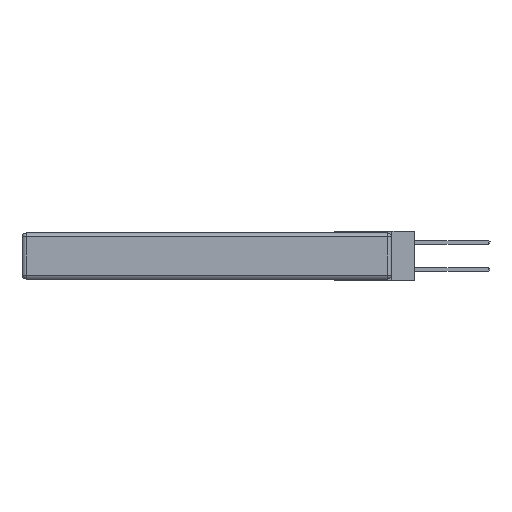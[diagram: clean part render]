
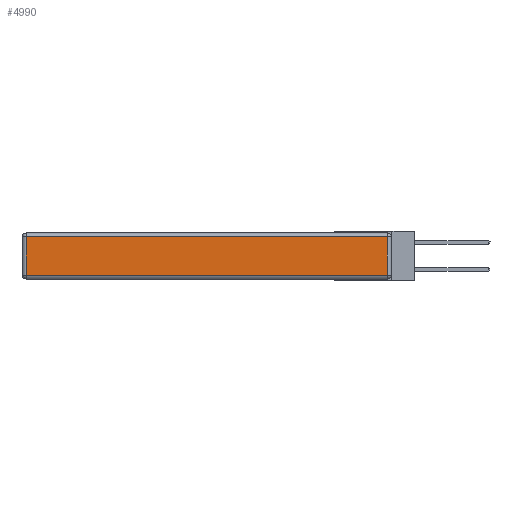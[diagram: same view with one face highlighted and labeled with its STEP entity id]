
A CAD part, left-side view. The second image highlights one B-rep face of the part: STEP entity #4990.
In plain terms, the highlighted planar face has unit normal (-1, 0, 0).
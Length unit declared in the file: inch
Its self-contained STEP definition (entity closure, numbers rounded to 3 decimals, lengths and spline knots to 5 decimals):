
#81 = CARTESIAN_POINT ( 'NONE',  ( 0., 0.03, -0.313 ) ) ;
#827 = AXIS2_PLACEMENT_3D ( 'NONE', #18220, #15513, #10340 ) ;
#891 = EDGE_CURVE ( 'NONE', #25712, #6162, #9175, .T. ) ;
#3154 = CARTESIAN_POINT ( 'NONE',  ( 0., 2.72, -0.313 ) ) ;
#4990 = ADVANCED_FACE ( 'NONE', ( #11364 ), #31747, .T. ) ;
#6085 = ORIENTED_EDGE ( 'NONE', *, *, #10357, .T. ) ;
#6162 = VERTEX_POINT ( 'NONE', #3154 ) ;
#9175 = LINE ( 'NONE', #9479, #23896 ) ;
#9393 = VERTEX_POINT ( 'NONE', #28363 ) ;
#9479 = CARTESIAN_POINT ( 'NONE',  ( 0., 2.72, -0.343 ) ) ;
#10340 = DIRECTION ( 'NONE',  ( 0., 0., 1. ) ) ;
#10357 = EDGE_CURVE ( 'NONE', #28477, #9393, #33723, .T. ) ;
#10739 = DIRECTION ( 'NONE',  ( 0., -1., 0. ) ) ;
#11364 = FACE_OUTER_BOUND ( 'NONE', #14737, .T. ) ;
#13096 = VECTOR ( 'NONE', #14843, 39.37008 ) ;
#13174 = CARTESIAN_POINT ( 'NONE',  ( 0., 2.72, -0.03 ) ) ;
#14737 = EDGE_LOOP ( 'NONE', ( #21364, #6085, #18728, #20100 ) ) ;
#14843 = DIRECTION ( 'NONE',  ( 0., 1., 0. ) ) ;
#14910 = DIRECTION ( 'NONE',  ( 0., 0., 1. ) ) ;
#15074 = VECTOR ( 'NONE', #10739, 39.37008 ) ;
#15513 = DIRECTION ( 'NONE',  ( -1., 0., 0. ) ) ;
#16770 = LINE ( 'NONE', #32406, #15074 ) ;
#18118 = VECTOR ( 'NONE', #14910, 39.37008 ) ;
#18220 = CARTESIAN_POINT ( 'NONE',  ( 0., 0., -0.343 ) ) ;
#18728 = ORIENTED_EDGE ( 'NONE', *, *, #25355, .T. ) ;
#20100 = ORIENTED_EDGE ( 'NONE', *, *, #891, .T. ) ;
#21364 = ORIENTED_EDGE ( 'NONE', *, *, #21480, .T. ) ;
#21480 = EDGE_CURVE ( 'NONE', #6162, #28477, #16770, .T. ) ;
#23896 = VECTOR ( 'NONE', #28061, 39.37008 ) ;
#25355 = EDGE_CURVE ( 'NONE', #9393, #25712, #27821, .T. ) ;
#25712 = VERTEX_POINT ( 'NONE', #13174 ) ;
#27821 = LINE ( 'NONE', #30753, #13096 ) ;
#28061 = DIRECTION ( 'NONE',  ( 0., 0., -1. ) ) ;
#28363 = CARTESIAN_POINT ( 'NONE',  ( 0., 0.03, -0.03 ) ) ;
#28477 = VERTEX_POINT ( 'NONE', #81 ) ;
#30753 = CARTESIAN_POINT ( 'NONE',  ( 0., 2.75, -0.03 ) ) ;
#31163 = CARTESIAN_POINT ( 'NONE',  ( 0., 0.03, -0.343 ) ) ;
#31747 = PLANE ( 'NONE',  #827 ) ;
#32406 = CARTESIAN_POINT ( 'NONE',  ( 0., 0., -0.313 ) ) ;
#33723 = LINE ( 'NONE', #31163, #18118 ) ;
